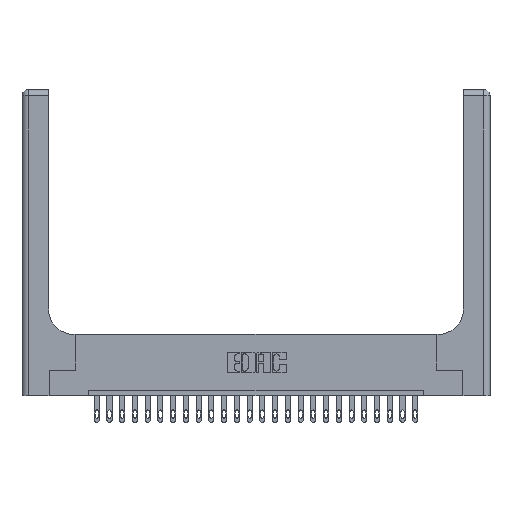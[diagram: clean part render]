
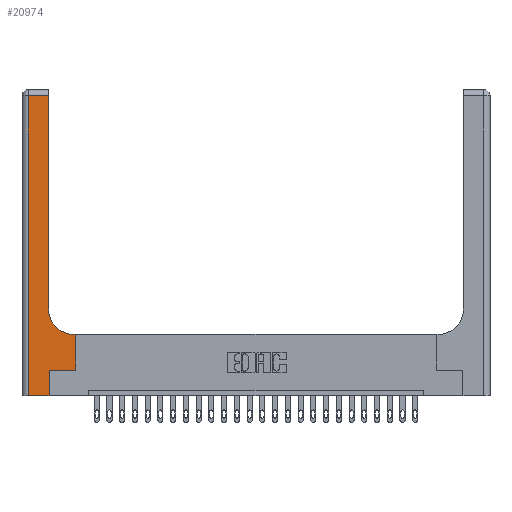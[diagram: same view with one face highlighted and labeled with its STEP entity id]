
A CAD part, top view. The second image highlights one B-rep face of the part: STEP entity #20974.
In plain terms, the highlighted planar face has unit normal (0, 0, 1).
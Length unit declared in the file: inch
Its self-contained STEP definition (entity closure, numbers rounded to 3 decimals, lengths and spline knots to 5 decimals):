
#120 = EDGE_CURVE ( 'NONE', #18881, #23067, #11896, .T. ) ;
#432 = ORIENTED_EDGE ( 'NONE', *, *, #19162, .T. ) ;
#1263 = CARTESIAN_POINT ( 'NONE',  ( 0.06, 0., 0.37 ) ) ;
#1632 = CIRCLE ( 'NONE', #23595, 0.25 ) ;
#2744 = CARTESIAN_POINT ( 'NONE',  ( 0.528, 0.25, 0.37 ) ) ;
#3142 = EDGE_CURVE ( 'NONE', #23067, #20443, #14242, .T. ) ;
#3413 = CARTESIAN_POINT ( 'NONE',  ( 0., 2.94, 0.37 ) ) ;
#3509 = VECTOR ( 'NONE', #15180, 39.37008 ) ;
#3532 = DIRECTION ( 'NONE',  ( -1., 0., 0. ) ) ;
#3807 = DIRECTION ( 'NONE',  ( 0., -1., 0. ) ) ;
#4002 = CARTESIAN_POINT ( 'NONE',  ( 0.26, 3., 0.37 ) ) ;
#4338 = CARTESIAN_POINT ( 'NONE',  ( 0., 3., 0.37 ) ) ;
#4457 = DIRECTION ( 'NONE',  ( 0., 0., -1. ) ) ;
#4584 = FACE_OUTER_BOUND ( 'NONE', #20473, .T. ) ;
#4923 = CARTESIAN_POINT ( 'NONE',  ( 0.51, 0.85, 0.37 ) ) ;
#5385 = CARTESIAN_POINT ( 'NONE',  ( 0.06, 3., 0.37 ) ) ;
#5538 = VERTEX_POINT ( 'NONE', #7218 ) ;
#6967 = VERTEX_POINT ( 'NONE', #9624 ) ;
#7218 = CARTESIAN_POINT ( 'NONE',  ( 0.265, 0.25, 0.37 ) ) ;
#7403 = DIRECTION ( 'NONE',  ( 1., 0., 0. ) ) ;
#7444 = VECTOR ( 'NONE', #7403, 39.37008 ) ;
#7601 = LINE ( 'NONE', #18589, #3509 ) ;
#7971 = VECTOR ( 'NONE', #19055, 39.37008 ) ;
#8574 = VECTOR ( 'NONE', #23210, 39.37008 ) ;
#8643 = DIRECTION ( 'NONE',  ( 1., 0., 0. ) ) ;
#9068 = CARTESIAN_POINT ( 'NONE',  ( 0.265, 0., 0.37 ) ) ;
#9237 = ORIENTED_EDGE ( 'NONE', *, *, #14786, .T. ) ;
#9624 = CARTESIAN_POINT ( 'NONE',  ( 0.26, 2.94, 0.37 ) ) ;
#9793 = CARTESIAN_POINT ( 'NONE',  ( 0.528, 0.25, 0.37 ) ) ;
#10075 = DIRECTION ( 'NONE',  ( 0., 1., 0. ) ) ;
#10492 = VECTOR ( 'NONE', #16409, 39.37008 ) ;
#10501 = CARTESIAN_POINT ( 'NONE',  ( 0.26, 0.85, 0.37 ) ) ;
#10800 = LINE ( 'NONE', #5385, #23348 ) ;
#10808 = DIRECTION ( 'NONE',  ( 0., 0., -1. ) ) ;
#11336 = LINE ( 'NONE', #4002, #10492 ) ;
#11427 = EDGE_CURVE ( 'NONE', #5538, #18881, #7601, .T. ) ;
#11673 = DIRECTION ( 'NONE',  ( -1., 0., 0. ) ) ;
#11692 = LINE ( 'NONE', #13614, #7971 ) ;
#11896 = LINE ( 'NONE', #2744, #22568 ) ;
#12367 = VERTEX_POINT ( 'NONE', #1263 ) ;
#13154 = VERTEX_POINT ( 'NONE', #16261 ) ;
#13614 = CARTESIAN_POINT ( 'NONE',  ( 0.265, 0., 0.37 ) ) ;
#14242 = LINE ( 'NONE', #14359, #20101 ) ;
#14359 = CARTESIAN_POINT ( 'NONE',  ( 0.26, 0.6, 0.37 ) ) ;
#14596 = ORIENTED_EDGE ( 'NONE', *, *, #3142, .T. ) ;
#14786 = EDGE_CURVE ( 'NONE', #20443, #19075, #1632, .T. ) ;
#14827 = ORIENTED_EDGE ( 'NONE', *, *, #15418, .T. ) ;
#15180 = DIRECTION ( 'NONE',  ( 1., 0., 0. ) ) ;
#15272 = PLANE ( 'NONE',  #16455 ) ;
#15418 = EDGE_CURVE ( 'NONE', #6967, #13154, #18109, .T. ) ;
#15591 = EDGE_CURVE ( 'NONE', #19075, #6967, #11336, .T. ) ;
#15673 = ORIENTED_EDGE ( 'NONE', *, *, #120, .T. ) ;
#16261 = CARTESIAN_POINT ( 'NONE',  ( 0.06, 2.94, 0.37 ) ) ;
#16311 = EDGE_CURVE ( 'NONE', #12367, #18708, #17050, .T. ) ;
#16409 = DIRECTION ( 'NONE',  ( 0., 1., 0. ) ) ;
#16455 = AXIS2_PLACEMENT_3D ( 'NONE', #4338, #4457, #11673 ) ;
#17050 = LINE ( 'NONE', #22249, #7444 ) ;
#17393 = EDGE_CURVE ( 'NONE', #13154, #12367, #10800, .T. ) ;
#17492 = CARTESIAN_POINT ( 'NONE',  ( 0.51, 0.6, 0.37 ) ) ;
#18055 = ORIENTED_EDGE ( 'NONE', *, *, #16311, .T. ) ;
#18109 = LINE ( 'NONE', #3413, #8574 ) ;
#18589 = CARTESIAN_POINT ( 'NONE',  ( 0.265, 0.25, 0.37 ) ) ;
#18653 = ORIENTED_EDGE ( 'NONE', *, *, #11427, .T. ) ;
#18708 = VERTEX_POINT ( 'NONE', #9068 ) ;
#18881 = VERTEX_POINT ( 'NONE', #9793 ) ;
#19055 = DIRECTION ( 'NONE',  ( 0., 1., 0. ) ) ;
#19075 = VERTEX_POINT ( 'NONE', #10501 ) ;
#19162 = EDGE_CURVE ( 'NONE', #18708, #5538, #11692, .T. ) ;
#19225 = CARTESIAN_POINT ( 'NONE',  ( 0.528, 0.6, 0.37 ) ) ;
#20101 = VECTOR ( 'NONE', #3532, 39.37008 ) ;
#20208 = ORIENTED_EDGE ( 'NONE', *, *, #17393, .T. ) ;
#20443 = VERTEX_POINT ( 'NONE', #17492 ) ;
#20473 = EDGE_LOOP ( 'NONE', ( #20709, #14827, #20208, #18055, #432, #18653, #15673, #14596, #9237 ) ) ;
#20709 = ORIENTED_EDGE ( 'NONE', *, *, #15591, .T. ) ;
#20974 = ADVANCED_FACE ( 'NONE', ( #4584 ), #15272, .F. ) ;
#22249 = CARTESIAN_POINT ( 'NONE',  ( 0., 0., 0.37 ) ) ;
#22568 = VECTOR ( 'NONE', #10075, 39.37008 ) ;
#23067 = VERTEX_POINT ( 'NONE', #19225 ) ;
#23210 = DIRECTION ( 'NONE',  ( -1., 0., 0. ) ) ;
#23348 = VECTOR ( 'NONE', #3807, 39.37008 ) ;
#23595 = AXIS2_PLACEMENT_3D ( 'NONE', #4923, #10808, #8643 ) ;
